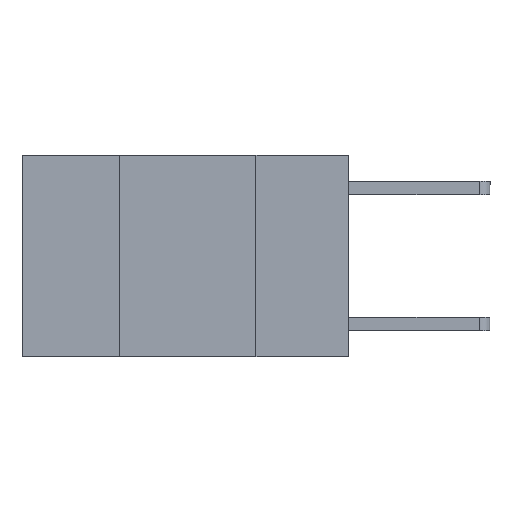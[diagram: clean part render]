
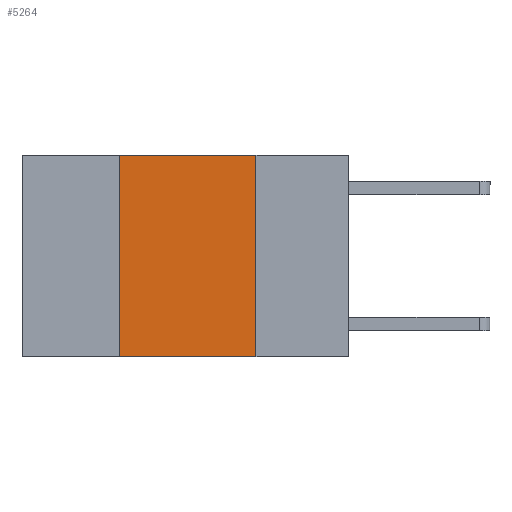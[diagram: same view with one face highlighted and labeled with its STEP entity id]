
A CAD part, left-side view. The second image highlights one B-rep face of the part: STEP entity #5264.
In plain terms, the highlighted planar face has unit normal (-1, 0, 0).
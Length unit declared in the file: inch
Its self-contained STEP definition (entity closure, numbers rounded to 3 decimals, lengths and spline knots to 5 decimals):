
#72 = PLANE ( 'NONE',  #7607 ) ;
#84 = ORIENTED_EDGE ( 'NONE', *, *, #5175, .F. ) ;
#119 = LINE ( 'NONE', #6745, #6670 ) ;
#1078 = EDGE_LOOP ( 'NONE', ( #8557, #84, #2773, #3518 ) ) ;
#1476 = EDGE_CURVE ( 'NONE', #6232, #6041, #6991, .T. ) ;
#1727 = CARTESIAN_POINT ( 'NONE',  ( 0., 0.17, 0. ) ) ;
#2054 = LINE ( 'NONE', #8538, #7141 ) ;
#2245 = DIRECTION ( 'NONE',  ( 0., 0., 1. ) ) ;
#2300 = FACE_OUTER_BOUND ( 'NONE', #1078, .T. ) ;
#2773 = ORIENTED_EDGE ( 'NONE', *, *, #5369, .F. ) ;
#3060 = DIRECTION ( 'NONE',  ( 1., 0., 0. ) ) ;
#3099 = LINE ( 'NONE', #8964, #8866 ) ;
#3518 = ORIENTED_EDGE ( 'NONE', *, *, #8454, .T. ) ;
#3597 = CARTESIAN_POINT ( 'NONE',  ( 0., 0.17, -0.37 ) ) ;
#3992 = VERTEX_POINT ( 'NONE', #4720 ) ;
#4191 = VECTOR ( 'NONE', #9176, 39.37008 ) ;
#4589 = DIRECTION ( 'NONE',  ( 0., -1., 0. ) ) ;
#4720 = CARTESIAN_POINT ( 'NONE',  ( 0., 0.42, 0. ) ) ;
#5116 = CARTESIAN_POINT ( 'NONE',  ( 0., 0.42, -0.37 ) ) ;
#5175 = EDGE_CURVE ( 'NONE', #3992, #6232, #2054, .T. ) ;
#5264 = ADVANCED_FACE ( 'NONE', ( #2300 ), #72, .F. ) ;
#5369 = EDGE_CURVE ( 'NONE', #8282, #3992, #119, .T. ) ;
#5938 = DIRECTION ( 'NONE',  ( 0., 0., -1. ) ) ;
#6022 = CARTESIAN_POINT ( 'NONE',  ( 0., 0.6, 0. ) ) ;
#6041 = VERTEX_POINT ( 'NONE', #3597 ) ;
#6232 = VERTEX_POINT ( 'NONE', #1727 ) ;
#6365 = CARTESIAN_POINT ( 'NONE',  ( 0., 0.17, 0. ) ) ;
#6670 = VECTOR ( 'NONE', #2245, 39.37008 ) ;
#6745 = CARTESIAN_POINT ( 'NONE',  ( 0., 0.42, 0. ) ) ;
#6991 = LINE ( 'NONE', #6365, #4191 ) ;
#7141 = VECTOR ( 'NONE', #7901, 39.37008 ) ;
#7607 = AXIS2_PLACEMENT_3D ( 'NONE', #6022, #3060, #5938 ) ;
#7901 = DIRECTION ( 'NONE',  ( 0., -1., 0. ) ) ;
#8282 = VERTEX_POINT ( 'NONE', #5116 ) ;
#8454 = EDGE_CURVE ( 'NONE', #8282, #6041, #3099, .T. ) ;
#8538 = CARTESIAN_POINT ( 'NONE',  ( 0., 0.6, 0. ) ) ;
#8557 = ORIENTED_EDGE ( 'NONE', *, *, #1476, .F. ) ;
#8866 = VECTOR ( 'NONE', #4589, 39.37008 ) ;
#8964 = CARTESIAN_POINT ( 'NONE',  ( 0., 0.6, -0.37 ) ) ;
#9176 = DIRECTION ( 'NONE',  ( 0., 0., -1. ) ) ;
